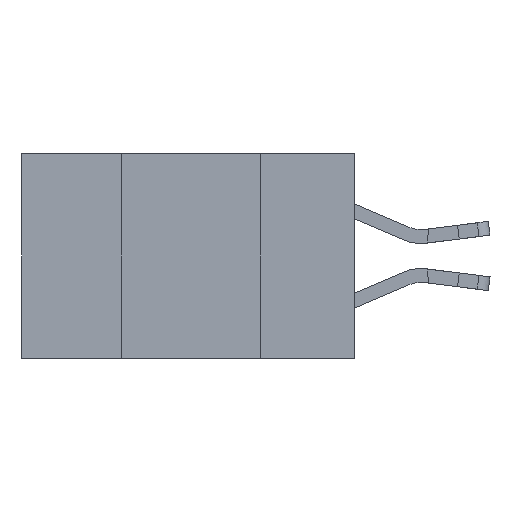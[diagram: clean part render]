
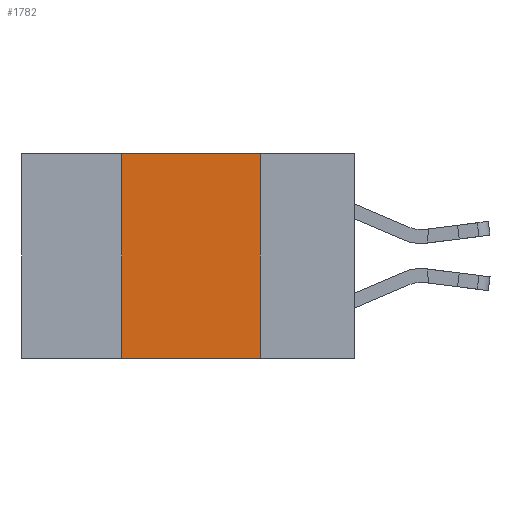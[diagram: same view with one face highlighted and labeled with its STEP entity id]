
A CAD part, left-side view. The second image highlights one B-rep face of the part: STEP entity #1782.
In plain terms, the highlighted planar face has unit normal (-1, 0, 0).
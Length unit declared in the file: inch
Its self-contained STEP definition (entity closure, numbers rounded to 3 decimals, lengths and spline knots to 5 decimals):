
#163 = LINE ( 'NONE', #8953, #798 ) ;
#287 = ORIENTED_EDGE ( 'NONE', *, *, #14406, .F. ) ;
#524 = EDGE_CURVE ( 'NONE', #16017, #4519, #163, .T. ) ;
#798 = VECTOR ( 'NONE', #872, 39.37008 ) ;
#872 = DIRECTION ( 'NONE',  ( 0., -1., 0. ) ) ;
#1379 = VECTOR ( 'NONE', #6847, 39.37008 ) ;
#1782 = ADVANCED_FACE ( 'NONE', ( #17178 ), #17280, .F. ) ;
#2054 = CARTESIAN_POINT ( 'NONE',  ( 0., 0.17, 0. ) ) ;
#2280 = LINE ( 'NONE', #9265, #9637 ) ;
#4421 = EDGE_CURVE ( 'NONE', #8542, #4519, #9395, .T. ) ;
#4519 = VERTEX_POINT ( 'NONE', #12778 ) ;
#5054 = DIRECTION ( 'NONE',  ( 0., 0., -1. ) ) ;
#5350 = CARTESIAN_POINT ( 'NONE',  ( 0., 0.42, 0. ) ) ;
#5478 = CARTESIAN_POINT ( 'NONE',  ( 0., 0.17, 0. ) ) ;
#5639 = CARTESIAN_POINT ( 'NONE',  ( 0., 0.42, -0.37 ) ) ;
#5907 = VECTOR ( 'NONE', #11110, 39.37008 ) ;
#6847 = DIRECTION ( 'NONE',  ( 0., 0., -1. ) ) ;
#7742 = VERTEX_POINT ( 'NONE', #5350 ) ;
#8542 = VERTEX_POINT ( 'NONE', #2054 ) ;
#8953 = CARTESIAN_POINT ( 'NONE',  ( 0., 0.6, -0.37 ) ) ;
#9043 = DIRECTION ( 'NONE',  ( 0., -1., 0. ) ) ;
#9265 = CARTESIAN_POINT ( 'NONE',  ( 0., 0.6, 0. ) ) ;
#9395 = LINE ( 'NONE', #5478, #1379 ) ;
#9637 = VECTOR ( 'NONE', #9043, 39.37008 ) ;
#10146 = LINE ( 'NONE', #13833, #5907 ) ;
#10292 = AXIS2_PLACEMENT_3D ( 'NONE', #14661, #13222, #5054 ) ;
#10435 = ORIENTED_EDGE ( 'NONE', *, *, #10930, .F. ) ;
#10930 = EDGE_CURVE ( 'NONE', #16017, #7742, #10146, .T. ) ;
#11110 = DIRECTION ( 'NONE',  ( 0., 0., 1. ) ) ;
#12778 = CARTESIAN_POINT ( 'NONE',  ( 0., 0.17, -0.37 ) ) ;
#13222 = DIRECTION ( 'NONE',  ( 1., 0., 0. ) ) ;
#13833 = CARTESIAN_POINT ( 'NONE',  ( 0., 0.42, 0. ) ) ;
#13856 = EDGE_LOOP ( 'NONE', ( #15548, #287, #10435, #14681 ) ) ;
#14406 = EDGE_CURVE ( 'NONE', #7742, #8542, #2280, .T. ) ;
#14661 = CARTESIAN_POINT ( 'NONE',  ( 0., 0.6, 0. ) ) ;
#14681 = ORIENTED_EDGE ( 'NONE', *, *, #524, .T. ) ;
#15548 = ORIENTED_EDGE ( 'NONE', *, *, #4421, .F. ) ;
#16017 = VERTEX_POINT ( 'NONE', #5639 ) ;
#17178 = FACE_OUTER_BOUND ( 'NONE', #13856, .T. ) ;
#17280 = PLANE ( 'NONE',  #10292 ) ;
